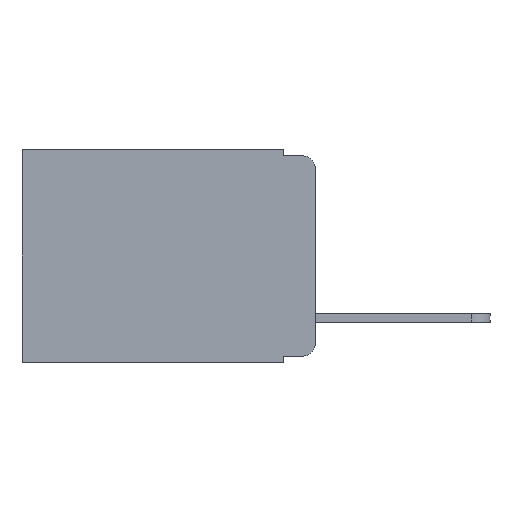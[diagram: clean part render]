
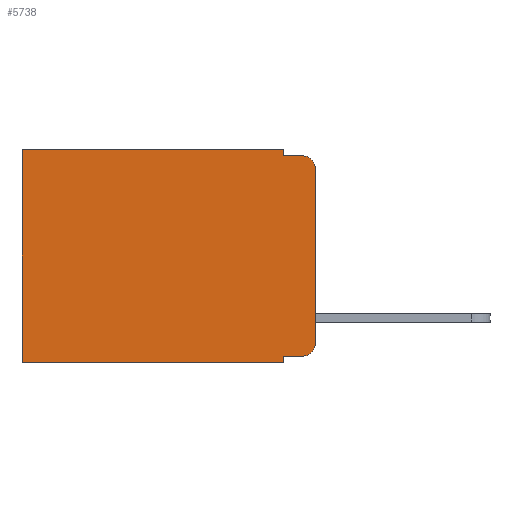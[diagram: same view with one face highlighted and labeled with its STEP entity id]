
A CAD part, left-side view. The second image highlights one B-rep face of the part: STEP entity #5738.
In plain terms, the highlighted planar face has unit normal (-1, 0, 0).
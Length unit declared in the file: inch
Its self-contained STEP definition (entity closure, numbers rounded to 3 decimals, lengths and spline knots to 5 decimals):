
#24 = CARTESIAN_POINT ( 'NONE',  ( 0.298, 0.051, -0.333 ) ) ;
#54 = VECTOR ( 'NONE', #4072, 39.37008 ) ;
#112 = ORIENTED_EDGE ( 'NONE', *, *, #5141, .F. ) ;
#142 = CARTESIAN_POINT ( 'NONE',  ( 0.298, 0.02, -0.03 ) ) ;
#230 = LINE ( 'NONE', #4740, #7510 ) ;
#299 = EDGE_CURVE ( 'NONE', #7584, #5868, #3862, .T. ) ;
#312 = ORIENTED_EDGE ( 'NONE', *, *, #5600, .F. ) ;
#557 = VERTEX_POINT ( 'NONE', #7008 ) ;
#565 = ORIENTED_EDGE ( 'NONE', *, *, #7385, .T. ) ;
#584 = DIRECTION ( 'NONE',  ( -1., 0., 0. ) ) ;
#715 = CARTESIAN_POINT ( 'NONE',  ( 0.298, 0.051, -0.01 ) ) ;
#776 = VECTOR ( 'NONE', #2797, 39.37008 ) ;
#847 = DIRECTION ( 'NONE',  ( 0., 0., -1. ) ) ;
#874 = EDGE_CURVE ( 'NONE', #7865, #6729, #4627, .T. ) ;
#1226 = VECTOR ( 'NONE', #2803, 39.37008 ) ;
#1351 = CARTESIAN_POINT ( 'NONE',  ( 0.298, 0.051, -0.333 ) ) ;
#1358 = CARTESIAN_POINT ( 'NONE',  ( 0.298, 0.051, 0. ) ) ;
#1458 = VERTEX_POINT ( 'NONE', #7987 ) ;
#1590 = CARTESIAN_POINT ( 'NONE',  ( 0.298, 0., -0.343 ) ) ;
#1804 = EDGE_LOOP ( 'NONE', ( #4317, #5694, #4650, #7414, #5043, #6754, #112, #312, #5662, #565 ) ) ;
#2212 = VECTOR ( 'NONE', #5186, 39.37008 ) ;
#2269 = VECTOR ( 'NONE', #7907, 39.37008 ) ;
#2370 = VERTEX_POINT ( 'NONE', #24 ) ;
#2372 = CARTESIAN_POINT ( 'NONE',  ( 0.298, 0., 0. ) ) ;
#2475 = VECTOR ( 'NONE', #7027, 39.37008 ) ;
#2482 = EDGE_CURVE ( 'NONE', #7865, #1458, #7218, .T. ) ;
#2656 = LINE ( 'NONE', #1351, #776 ) ;
#2797 = DIRECTION ( 'NONE',  ( 0., -1., 0. ) ) ;
#2803 = DIRECTION ( 'NONE',  ( 0., 0., -1. ) ) ;
#2806 = FACE_OUTER_BOUND ( 'NONE', #1804, .T. ) ;
#3024 = VERTEX_POINT ( 'NONE', #715 ) ;
#3332 = AXIS2_PLACEMENT_3D ( 'NONE', #142, #5070, #847 ) ;
#3789 = DIRECTION ( 'NONE',  ( 1., 0., 0. ) ) ;
#3862 = LINE ( 'NONE', #5891, #2212 ) ;
#3946 = CARTESIAN_POINT ( 'NONE',  ( 0.298, 0., -0.03 ) ) ;
#4072 = DIRECTION ( 'NONE',  ( 0., 0., -1. ) ) ;
#4317 = ORIENTED_EDGE ( 'NONE', *, *, #874, .F. ) ;
#4327 = CARTESIAN_POINT ( 'NONE',  ( 0.298, 0.051, 0. ) ) ;
#4471 = VERTEX_POINT ( 'NONE', #5508 ) ;
#4627 = LINE ( 'NONE', #8079, #8122 ) ;
#4646 = CARTESIAN_POINT ( 'NONE',  ( 0.298, 0.473, 0. ) ) ;
#4650 = ORIENTED_EDGE ( 'NONE', *, *, #7134, .F. ) ;
#4740 = CARTESIAN_POINT ( 'NONE',  ( 0.298, 0.051, -0.01 ) ) ;
#4821 = CARTESIAN_POINT ( 'NONE',  ( 0.298, 0.02, -0.313 ) ) ;
#4984 = LINE ( 'NONE', #1358, #1226 ) ;
#5043 = ORIENTED_EDGE ( 'NONE', *, *, #299, .T. ) ;
#5070 = DIRECTION ( 'NONE',  ( -1., 0., 0. ) ) ;
#5141 = EDGE_CURVE ( 'NONE', #4471, #7498, #6004, .T. ) ;
#5177 = PLANE ( 'NONE',  #5282 ) ;
#5186 = DIRECTION ( 'NONE',  ( 0., 1., 0. ) ) ;
#5282 = AXIS2_PLACEMENT_3D ( 'NONE', #2372, #3789, #8695 ) ;
#5441 = DIRECTION ( 'NONE',  ( 0., -1., 0. ) ) ;
#5478 = EDGE_CURVE ( 'NONE', #5868, #7498, #6887, .T. ) ;
#5508 = CARTESIAN_POINT ( 'NONE',  ( 0.298, 0.051, -0.343 ) ) ;
#5521 = DIRECTION ( 'NONE',  ( 0., 0., -1. ) ) ;
#5600 = EDGE_CURVE ( 'NONE', #2370, #4471, #6218, .T. ) ;
#5608 = CARTESIAN_POINT ( 'NONE',  ( 0.298, 0.051, 0. ) ) ;
#5662 = ORIENTED_EDGE ( 'NONE', *, *, #7270, .T. ) ;
#5694 = ORIENTED_EDGE ( 'NONE', *, *, #2482, .T. ) ;
#5738 = ADVANCED_FACE ( 'NONE', ( #2806 ), #5177, .F. ) ;
#5868 = VERTEX_POINT ( 'NONE', #4646 ) ;
#5891 = CARTESIAN_POINT ( 'NONE',  ( 0.298, 0., 0. ) ) ;
#6004 = LINE ( 'NONE', #1590, #2269 ) ;
#6218 = LINE ( 'NONE', #5608, #2475 ) ;
#6729 = VERTEX_POINT ( 'NONE', #7665 ) ;
#6754 = ORIENTED_EDGE ( 'NONE', *, *, #5478, .T. ) ;
#6764 = EDGE_CURVE ( 'NONE', #7584, #3024, #4984, .T. ) ;
#6887 = LINE ( 'NONE', #8260, #54 ) ;
#7008 = CARTESIAN_POINT ( 'NONE',  ( 0.298, 0.02, -0.333 ) ) ;
#7027 = DIRECTION ( 'NONE',  ( 0., 0., -1. ) ) ;
#7036 = CARTESIAN_POINT ( 'NONE',  ( 0.298, 0.473, -0.343 ) ) ;
#7134 = EDGE_CURVE ( 'NONE', #3024, #1458, #230, .T. ) ;
#7218 = CIRCLE ( 'NONE', #3332, 0.02 ) ;
#7270 = EDGE_CURVE ( 'NONE', #2370, #557, #2656, .T. ) ;
#7385 = EDGE_CURVE ( 'NONE', #557, #6729, #9028, .T. ) ;
#7414 = ORIENTED_EDGE ( 'NONE', *, *, #6764, .F. ) ;
#7498 = VERTEX_POINT ( 'NONE', #7036 ) ;
#7510 = VECTOR ( 'NONE', #5441, 39.37008 ) ;
#7584 = VERTEX_POINT ( 'NONE', #4327 ) ;
#7665 = CARTESIAN_POINT ( 'NONE',  ( 0.298, 0., -0.313 ) ) ;
#7865 = VERTEX_POINT ( 'NONE', #3946 ) ;
#7907 = DIRECTION ( 'NONE',  ( 0., 1., 0. ) ) ;
#7987 = CARTESIAN_POINT ( 'NONE',  ( 0.298, 0.02, -0.01 ) ) ;
#8079 = CARTESIAN_POINT ( 'NONE',  ( 0.298, 0., 0. ) ) ;
#8122 = VECTOR ( 'NONE', #8789, 39.37008 ) ;
#8260 = CARTESIAN_POINT ( 'NONE',  ( 0.298, 0.473, 0. ) ) ;
#8695 = DIRECTION ( 'NONE',  ( 0., 0., -1. ) ) ;
#8789 = DIRECTION ( 'NONE',  ( 0., 0., -1. ) ) ;
#9028 = CIRCLE ( 'NONE', #9109, 0.02 ) ;
#9109 = AXIS2_PLACEMENT_3D ( 'NONE', #4821, #584, #5521 ) ;
